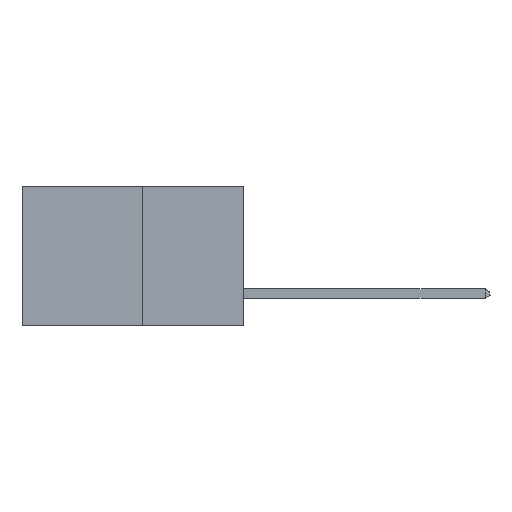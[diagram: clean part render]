
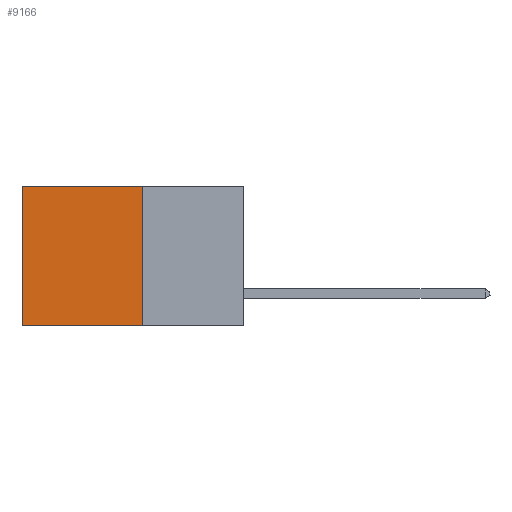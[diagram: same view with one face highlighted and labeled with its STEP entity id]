
A CAD part, left-side view. The second image highlights one B-rep face of the part: STEP entity #9166.
In plain terms, the highlighted planar face has unit normal (-1, 0, 0).
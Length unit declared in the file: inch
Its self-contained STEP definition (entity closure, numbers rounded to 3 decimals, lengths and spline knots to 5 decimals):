
#835 = EDGE_CURVE ( 'NONE', #24565, #6984, #23738, .T. ) ;
#1033 = CARTESIAN_POINT ( 'NONE',  ( 0.277, 0.27, -0.37 ) ) ;
#2404 = LINE ( 'NONE', #1033, #13176 ) ;
#3188 = CARTESIAN_POINT ( 'NONE',  ( 0.277, 0.27, -0.37 ) ) ;
#3210 = DIRECTION ( 'NONE',  ( 0., 1., 0. ) ) ;
#4055 = LINE ( 'NONE', #9560, #20455 ) ;
#4475 = ORIENTED_EDGE ( 'NONE', *, *, #25427, .F. ) ;
#5526 = CARTESIAN_POINT ( 'NONE',  ( 0.277, 0.27, 0. ) ) ;
#5563 = VERTEX_POINT ( 'NONE', #3188 ) ;
#6984 = VERTEX_POINT ( 'NONE', #20600 ) ;
#7343 = EDGE_LOOP ( 'NONE', ( #15488, #4475, #23705, #22295 ) ) ;
#8118 = FACE_OUTER_BOUND ( 'NONE', #7343, .T. ) ;
#8287 = CARTESIAN_POINT ( 'NONE',  ( 0.277, 0.27, -0.37 ) ) ;
#8298 = EDGE_CURVE ( 'NONE', #25120, #24565, #8839, .T. ) ;
#8839 = LINE ( 'NONE', #5526, #25227 ) ;
#9166 = ADVANCED_FACE ( 'NONE', ( #8118 ), #21082, .F. ) ;
#9560 = CARTESIAN_POINT ( 'NONE',  ( 0.277, 0.27, -0.37 ) ) ;
#10054 = AXIS2_PLACEMENT_3D ( 'NONE', #8287, #23202, #10434 ) ;
#10434 = DIRECTION ( 'NONE',  ( 0., 0., -1. ) ) ;
#13102 = VECTOR ( 'NONE', #22761, 39.37008 ) ;
#13176 = VECTOR ( 'NONE', #3210, 39.37008 ) ;
#14064 = DIRECTION ( 'NONE',  ( 0., 1., 0. ) ) ;
#15488 = ORIENTED_EDGE ( 'NONE', *, *, #835, .T. ) ;
#17961 = DIRECTION ( 'NONE',  ( 0., 0., -1. ) ) ;
#19128 = EDGE_CURVE ( 'NONE', #25120, #5563, #4055, .T. ) ;
#19136 = CARTESIAN_POINT ( 'NONE',  ( 0.277, 0.59, 0. ) ) ;
#20455 = VECTOR ( 'NONE', #17961, 39.37008 ) ;
#20600 = CARTESIAN_POINT ( 'NONE',  ( 0.277, 0.59, -0.37 ) ) ;
#21082 = PLANE ( 'NONE',  #10054 ) ;
#22295 = ORIENTED_EDGE ( 'NONE', *, *, #8298, .T. ) ;
#22761 = DIRECTION ( 'NONE',  ( 0., 0., -1. ) ) ;
#22930 = CARTESIAN_POINT ( 'NONE',  ( 0.277, 0.59, -0.37 ) ) ;
#23202 = DIRECTION ( 'NONE',  ( 1., 0., 0. ) ) ;
#23705 = ORIENTED_EDGE ( 'NONE', *, *, #19128, .F. ) ;
#23738 = LINE ( 'NONE', #22930, #13102 ) ;
#24565 = VERTEX_POINT ( 'NONE', #19136 ) ;
#25120 = VERTEX_POINT ( 'NONE', #25724 ) ;
#25227 = VECTOR ( 'NONE', #14064, 39.37008 ) ;
#25427 = EDGE_CURVE ( 'NONE', #5563, #6984, #2404, .T. ) ;
#25724 = CARTESIAN_POINT ( 'NONE',  ( 0.277, 0.27, 0. ) ) ;
